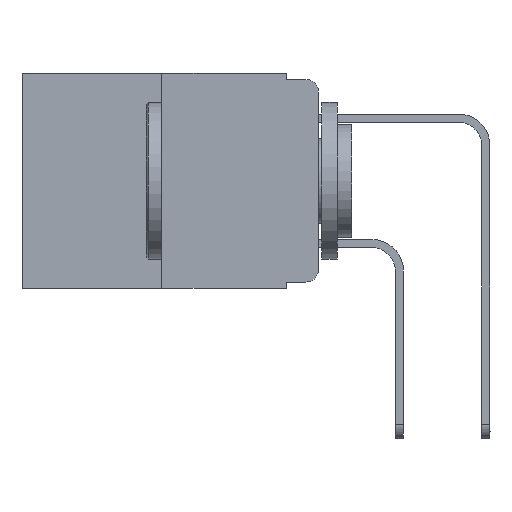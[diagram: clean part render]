
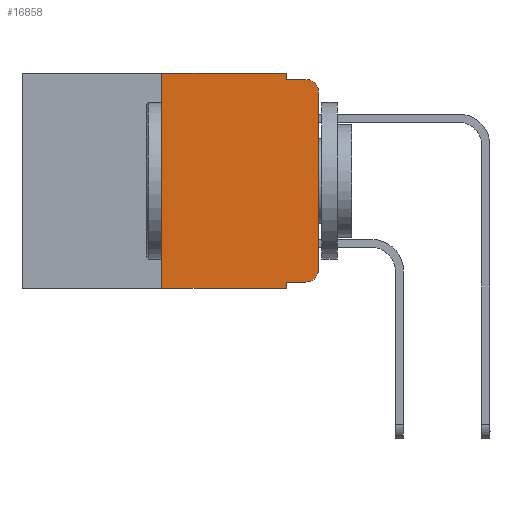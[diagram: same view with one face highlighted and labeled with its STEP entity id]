
A CAD part, left-side view. The second image highlights one B-rep face of the part: STEP entity #16858.
In plain terms, the highlighted planar face has unit normal (-1, 0, 0).
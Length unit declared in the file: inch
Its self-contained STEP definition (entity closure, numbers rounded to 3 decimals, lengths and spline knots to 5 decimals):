
#186 = CARTESIAN_POINT ( 'NONE',  ( 0., 0.051, 0. ) ) ;
#219 = EDGE_CURVE ( 'NONE', #1847, #8903, #2154, .T. ) ;
#679 = VECTOR ( 'NONE', #4555, 39.37008 ) ;
#942 = ORIENTED_EDGE ( 'NONE', *, *, #6232, .T. ) ;
#1334 = LINE ( 'NONE', #19207, #11896 ) ;
#1393 = DIRECTION ( 'NONE',  ( 1., 0., 0. ) ) ;
#1773 = ORIENTED_EDGE ( 'NONE', *, *, #8072, .F. ) ;
#1847 = VERTEX_POINT ( 'NONE', #10119 ) ;
#2050 = VERTEX_POINT ( 'NONE', #13519 ) ;
#2154 = LINE ( 'NONE', #3012, #679 ) ;
#2307 = EDGE_CURVE ( 'NONE', #1847, #10672, #8066, .T. ) ;
#2767 = ORIENTED_EDGE ( 'NONE', *, *, #18042, .T. ) ;
#2969 = ORIENTED_EDGE ( 'NONE', *, *, #11572, .F. ) ;
#3012 = CARTESIAN_POINT ( 'NONE',  ( 0., 0.25, 0. ) ) ;
#3080 = VERTEX_POINT ( 'NONE', #18636 ) ;
#3233 = DIRECTION ( 'NONE',  ( 0., 0., -1. ) ) ;
#3922 = CARTESIAN_POINT ( 'NONE',  ( 0., 0.25, 0. ) ) ;
#3928 = DIRECTION ( 'NONE',  ( 0., 0., -1. ) ) ;
#4477 = PLANE ( 'NONE',  #7265 ) ;
#4555 = DIRECTION ( 'NONE',  ( 0., 0., 1. ) ) ;
#4831 = LINE ( 'NONE', #6937, #15924 ) ;
#5364 = DIRECTION ( 'NONE',  ( 0., -1., 0. ) ) ;
#5484 = DIRECTION ( 'NONE',  ( -1., 0., 0. ) ) ;
#5878 = CARTESIAN_POINT ( 'NONE',  ( 0., 0.051, -0.343 ) ) ;
#5946 = LINE ( 'NONE', #7027, #7855 ) ;
#6141 = VECTOR ( 'NONE', #8990, 39.37008 ) ;
#6232 = EDGE_CURVE ( 'NONE', #2050, #6888, #15767, .T. ) ;
#6273 = VERTEX_POINT ( 'NONE', #13429 ) ;
#6740 = CARTESIAN_POINT ( 'NONE',  ( 0., 0., -0.03 ) ) ;
#6803 = ORIENTED_EDGE ( 'NONE', *, *, #10614, .T. ) ;
#6888 = VERTEX_POINT ( 'NONE', #6740 ) ;
#6937 = CARTESIAN_POINT ( 'NONE',  ( 0., 0.051, -0.01 ) ) ;
#7027 = CARTESIAN_POINT ( 'NONE',  ( 0., 0.051, -0.333 ) ) ;
#7061 = DIRECTION ( 'NONE',  ( 0., 0., -1. ) ) ;
#7153 = DIRECTION ( 'NONE',  ( 0., -1., 0. ) ) ;
#7265 = AXIS2_PLACEMENT_3D ( 'NONE', #13352, #1393, #8505 ) ;
#7855 = VECTOR ( 'NONE', #7153, 39.37008 ) ;
#8066 = LINE ( 'NONE', #15522, #12410 ) ;
#8072 = EDGE_CURVE ( 'NONE', #12423, #15543, #4831, .T. ) ;
#8505 = DIRECTION ( 'NONE',  ( 0., 0., -1. ) ) ;
#8637 = CARTESIAN_POINT ( 'NONE',  ( 0., 0.02, -0.01 ) ) ;
#8800 = CARTESIAN_POINT ( 'NONE',  ( 0., 0.473, 0. ) ) ;
#8834 = ORIENTED_EDGE ( 'NONE', *, *, #19741, .F. ) ;
#8903 = VERTEX_POINT ( 'NONE', #3922 ) ;
#8990 = DIRECTION ( 'NONE',  ( 0., 0., 1. ) ) ;
#9124 = ORIENTED_EDGE ( 'NONE', *, *, #219, .F. ) ;
#9445 = CARTESIAN_POINT ( 'NONE',  ( 0., 0.051, -0.333 ) ) ;
#10016 = EDGE_CURVE ( 'NONE', #8903, #3080, #13437, .T. ) ;
#10119 = CARTESIAN_POINT ( 'NONE',  ( 0., 0.25, -0.343 ) ) ;
#10614 = EDGE_CURVE ( 'NONE', #15725, #6273, #5946, .T. ) ;
#10672 = VERTEX_POINT ( 'NONE', #5878 ) ;
#10725 = FACE_OUTER_BOUND ( 'NONE', #16220, .T. ) ;
#11032 = CIRCLE ( 'NONE', #13970, 0.02 ) ;
#11572 = EDGE_CURVE ( 'NONE', #15725, #10672, #1334, .T. ) ;
#11896 = VECTOR ( 'NONE', #3928, 39.37008 ) ;
#11972 = CIRCLE ( 'NONE', #18498, 0.02 ) ;
#12018 = CARTESIAN_POINT ( 'NONE',  ( 0., 0., 0. ) ) ;
#12219 = DIRECTION ( 'NONE',  ( 0., -1., 0. ) ) ;
#12343 = DIRECTION ( 'NONE',  ( -1., 0., 0. ) ) ;
#12410 = VECTOR ( 'NONE', #12219, 39.37008 ) ;
#12423 = VERTEX_POINT ( 'NONE', #18464 ) ;
#13352 = CARTESIAN_POINT ( 'NONE',  ( 0., 0.473, 0. ) ) ;
#13429 = CARTESIAN_POINT ( 'NONE',  ( 0., 0.02, -0.333 ) ) ;
#13437 = LINE ( 'NONE', #8800, #16065 ) ;
#13519 = CARTESIAN_POINT ( 'NONE',  ( 0., 0., -0.313 ) ) ;
#13969 = DIRECTION ( 'NONE',  ( 0., 0., -1. ) ) ;
#13970 = AXIS2_PLACEMENT_3D ( 'NONE', #15574, #12343, #13969 ) ;
#14667 = ORIENTED_EDGE ( 'NONE', *, *, #2307, .T. ) ;
#14729 = CARTESIAN_POINT ( 'NONE',  ( 0., 0.02, -0.313 ) ) ;
#15522 = CARTESIAN_POINT ( 'NONE',  ( 0., 0.473, -0.343 ) ) ;
#15543 = VERTEX_POINT ( 'NONE', #8637 ) ;
#15574 = CARTESIAN_POINT ( 'NONE',  ( 0., 0.02, -0.03 ) ) ;
#15616 = ORIENTED_EDGE ( 'NONE', *, *, #10016, .F. ) ;
#15725 = VERTEX_POINT ( 'NONE', #9445 ) ;
#15745 = EDGE_CURVE ( 'NONE', #6888, #15543, #11032, .T. ) ;
#15767 = LINE ( 'NONE', #12018, #6141 ) ;
#15924 = VECTOR ( 'NONE', #5364, 39.37008 ) ;
#16065 = VECTOR ( 'NONE', #19572, 39.37008 ) ;
#16211 = LINE ( 'NONE', #186, #18640 ) ;
#16220 = EDGE_LOOP ( 'NONE', ( #942, #17384, #1773, #8834, #15616, #9124, #14667, #2969, #6803, #2767 ) ) ;
#16858 = ADVANCED_FACE ( 'NONE', ( #10725 ), #4477, .F. ) ;
#17384 = ORIENTED_EDGE ( 'NONE', *, *, #15745, .T. ) ;
#18042 = EDGE_CURVE ( 'NONE', #6273, #2050, #11972, .T. ) ;
#18464 = CARTESIAN_POINT ( 'NONE',  ( 0., 0.051, -0.01 ) ) ;
#18498 = AXIS2_PLACEMENT_3D ( 'NONE', #14729, #5484, #7061 ) ;
#18636 = CARTESIAN_POINT ( 'NONE',  ( 0., 0.051, 0. ) ) ;
#18640 = VECTOR ( 'NONE', #3233, 39.37008 ) ;
#19207 = CARTESIAN_POINT ( 'NONE',  ( 0., 0.051, 0. ) ) ;
#19572 = DIRECTION ( 'NONE',  ( 0., -1., 0. ) ) ;
#19741 = EDGE_CURVE ( 'NONE', #3080, #12423, #16211, .T. ) ;
